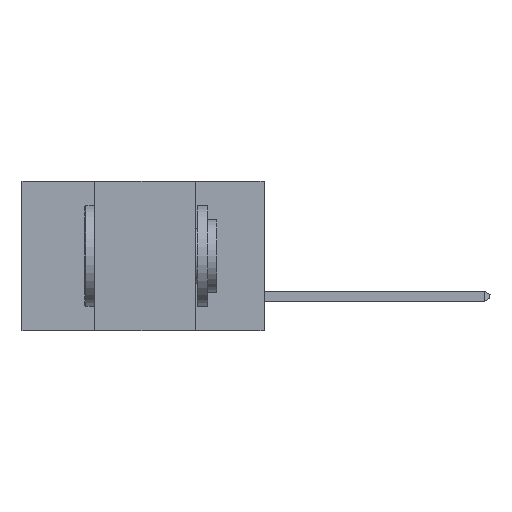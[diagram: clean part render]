
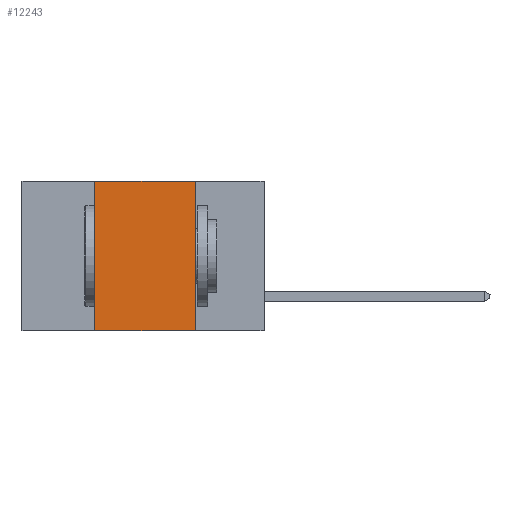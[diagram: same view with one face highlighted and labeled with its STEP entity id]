
A CAD part, left-side view. The second image highlights one B-rep face of the part: STEP entity #12243.
In plain terms, the highlighted planar face has unit normal (-1, 0, 0).
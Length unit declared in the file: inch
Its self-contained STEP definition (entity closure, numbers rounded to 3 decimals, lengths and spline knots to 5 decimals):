
#529 = DIRECTION ( 'NONE',  ( 0., -1., 0. ) ) ;
#1181 = DIRECTION ( 'NONE',  ( 1., 0., 0. ) ) ;
#1629 = EDGE_CURVE ( 'NONE', #9634, #12115, #2625, .T. ) ;
#1738 = VECTOR ( 'NONE', #5942, 39.37008 ) ;
#1783 = VECTOR ( 'NONE', #4401, 39.37008 ) ;
#2442 = VECTOR ( 'NONE', #529, 39.37008 ) ;
#2625 = LINE ( 'NONE', #10703, #9441 ) ;
#3146 = EDGE_CURVE ( 'NONE', #8031, #9634, #10445, .T. ) ;
#4009 = CARTESIAN_POINT ( 'NONE',  ( 0., 0.17, -0.37 ) ) ;
#4115 = CARTESIAN_POINT ( 'NONE',  ( 0., 0.42, -0.37 ) ) ;
#4263 = CARTESIAN_POINT ( 'NONE',  ( 0., 0.6, -0.37 ) ) ;
#4401 = DIRECTION ( 'NONE',  ( 0., -1., 0. ) ) ;
#4623 = ORIENTED_EDGE ( 'NONE', *, *, #4966, .F. ) ;
#4966 = EDGE_CURVE ( 'NONE', #12995, #8031, #11208, .T. ) ;
#5284 = FACE_OUTER_BOUND ( 'NONE', #10534, .T. ) ;
#5942 = DIRECTION ( 'NONE',  ( 0., 0., 1. ) ) ;
#6137 = CARTESIAN_POINT ( 'NONE',  ( 0., 0.42, -0.37 ) ) ;
#6221 = PLANE ( 'NONE',  #10441 ) ;
#6562 = ORIENTED_EDGE ( 'NONE', *, *, #3146, .F. ) ;
#6866 = CARTESIAN_POINT ( 'NONE',  ( 0., 0.17, 0. ) ) ;
#8031 = VERTEX_POINT ( 'NONE', #8518 ) ;
#8148 = CARTESIAN_POINT ( 'NONE',  ( 0., 0.6, 0. ) ) ;
#8341 = DIRECTION ( 'NONE',  ( 0., 0., -1. ) ) ;
#8518 = CARTESIAN_POINT ( 'NONE',  ( 0., 0.42, 0. ) ) ;
#9438 = EDGE_CURVE ( 'NONE', #12995, #12115, #11331, .T. ) ;
#9441 = VECTOR ( 'NONE', #9712, 39.37008 ) ;
#9634 = VERTEX_POINT ( 'NONE', #6866 ) ;
#9712 = DIRECTION ( 'NONE',  ( 0., 0., -1. ) ) ;
#9942 = ORIENTED_EDGE ( 'NONE', *, *, #9438, .T. ) ;
#10441 = AXIS2_PLACEMENT_3D ( 'NONE', #8148, #1181, #8341 ) ;
#10445 = LINE ( 'NONE', #12590, #2442 ) ;
#10534 = EDGE_LOOP ( 'NONE', ( #12230, #6562, #4623, #9942 ) ) ;
#10703 = CARTESIAN_POINT ( 'NONE',  ( 0., 0.17, -0.37 ) ) ;
#11208 = LINE ( 'NONE', #6137, #1738 ) ;
#11331 = LINE ( 'NONE', #4263, #1783 ) ;
#12115 = VERTEX_POINT ( 'NONE', #4009 ) ;
#12230 = ORIENTED_EDGE ( 'NONE', *, *, #1629, .F. ) ;
#12243 = ADVANCED_FACE ( 'NONE', ( #5284 ), #6221, .F. ) ;
#12590 = CARTESIAN_POINT ( 'NONE',  ( 0., 0.6, 0. ) ) ;
#12995 = VERTEX_POINT ( 'NONE', #4115 ) ;
